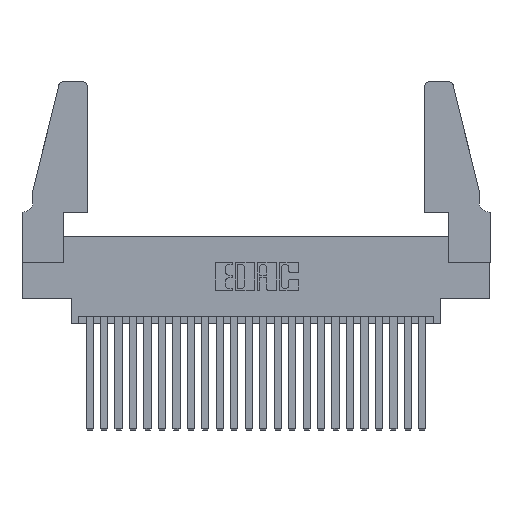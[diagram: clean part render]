
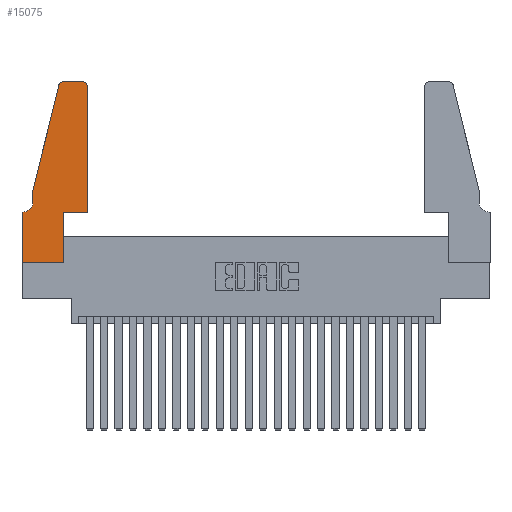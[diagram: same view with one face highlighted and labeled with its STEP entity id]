
A CAD part, top view. The second image highlights one B-rep face of the part: STEP entity #15075.
In plain terms, the highlighted planar face has unit normal (0, 0, 1).
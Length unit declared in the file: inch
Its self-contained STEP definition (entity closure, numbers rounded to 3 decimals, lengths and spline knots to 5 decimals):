
#36 = CARTESIAN_POINT ( 'NONE',  ( 0.2865, 0., 0.37 ) ) ;
#177 = CARTESIAN_POINT ( 'NONE',  ( 0.4505, 0.35, 0.37 ) ) ;
#179 = DIRECTION ( 'NONE',  ( 1., 0., 0. ) ) ;
#201 = VECTOR ( 'NONE', #4903, 39.37008 ) ;
#260 = DIRECTION ( 'NONE',  ( 0., 0., 1. ) ) ;
#274 = VECTOR ( 'NONE', #13782, 39.37008 ) ;
#281 = CARTESIAN_POINT ( 'NONE',  ( 0.2865, 0.35, 0.37 ) ) ;
#748 = CARTESIAN_POINT ( 'NONE',  ( 0.25487, 1.22718, 0.37 ) ) ;
#783 = EDGE_CURVE ( 'NONE', #15887, #18100, #9554, .T. ) ;
#803 = DIRECTION ( 'NONE',  ( -1., 0., 0. ) ) ;
#973 = VECTOR ( 'NONE', #17176, 39.37008 ) ;
#1058 = CARTESIAN_POINT ( 'NONE',  ( 0.0755, 0.42, 0.37 ) ) ;
#1167 = LINE ( 'NONE', #7243, #19781 ) ;
#1214 = CARTESIAN_POINT ( 'NONE',  ( 0.2865, 0.35, 0.37 ) ) ;
#1981 = ORIENTED_EDGE ( 'NONE', *, *, #14536, .T. ) ;
#2157 = LINE ( 'NONE', #17942, #21330 ) ;
#2161 = CARTESIAN_POINT ( 'NONE',  ( 0., 0., 0.37 ) ) ;
#2230 = CARTESIAN_POINT ( 'NONE',  ( 0., 0.35, 0.37 ) ) ;
#2284 = VERTEX_POINT ( 'NONE', #1058 ) ;
#2475 = ORIENTED_EDGE ( 'NONE', *, *, #21416, .T. ) ;
#2632 = DIRECTION ( 'NONE',  ( 0., 0., 1. ) ) ;
#2735 = CARTESIAN_POINT ( 'NONE',  ( 0.0755, 0.35, 0.37 ) ) ;
#2858 = EDGE_CURVE ( 'NONE', #8271, #17694, #12564, .T. ) ;
#2925 = DIRECTION ( 'NONE',  ( -1., 0., 0. ) ) ;
#2994 = ORIENTED_EDGE ( 'NONE', *, *, #15100, .T. ) ;
#3627 = CARTESIAN_POINT ( 'NONE',  ( 0.4205, 1.25, 0.37 ) ) ;
#3668 = DIRECTION ( 'NONE',  ( 0., -1., 0. ) ) ;
#3981 = CARTESIAN_POINT ( 'NONE',  ( 0.4505, 0.35, 0.37 ) ) ;
#4006 = ORIENTED_EDGE ( 'NONE', *, *, #16755, .T. ) ;
#4369 = LINE ( 'NONE', #20888, #9184 ) ;
#4506 = ORIENTED_EDGE ( 'NONE', *, *, #20100, .T. ) ;
#4723 = VERTEX_POINT ( 'NONE', #20505 ) ;
#4899 = LINE ( 'NONE', #2161, #13919 ) ;
#4903 = DIRECTION ( 'NONE',  ( 0., 1., 0. ) ) ;
#5334 = VECTOR ( 'NONE', #10659, 39.37008 ) ;
#5396 = PLANE ( 'NONE',  #8343 ) ;
#7199 = DIRECTION ( 'NONE',  ( 0., 0., 1. ) ) ;
#7243 = CARTESIAN_POINT ( 'NONE',  ( 0.0755, 0.5, 0.37 ) ) ;
#7480 = VERTEX_POINT ( 'NONE', #21115 ) ;
#7668 = DIRECTION ( 'NONE',  ( 1., 0., 0. ) ) ;
#8141 = ORIENTED_EDGE ( 'NONE', *, *, #18767, .T. ) ;
#8268 = VERTEX_POINT ( 'NONE', #281 ) ;
#8271 = VERTEX_POINT ( 'NONE', #9369 ) ;
#8343 = AXIS2_PLACEMENT_3D ( 'NONE', #12489, #7199, #19747 ) ;
#8562 = EDGE_CURVE ( 'NONE', #8845, #8271, #4369, .T. ) ;
#8845 = VERTEX_POINT ( 'NONE', #3627 ) ;
#9036 = CARTESIAN_POINT ( 'NONE',  ( 0.4505, 1.22, 0.37 ) ) ;
#9133 = EDGE_CURVE ( 'NONE', #2284, #7480, #18961, .T. ) ;
#9184 = VECTOR ( 'NONE', #2925, 39.37008 ) ;
#9369 = CARTESIAN_POINT ( 'NONE',  ( 0.284, 1.25, 0.37 ) ) ;
#9376 = ORIENTED_EDGE ( 'NONE', *, *, #783, .T. ) ;
#9554 = LINE ( 'NONE', #177, #5334 ) ;
#9665 = VERTEX_POINT ( 'NONE', #2230 ) ;
#10659 = DIRECTION ( 'NONE',  ( 0., 1., 0. ) ) ;
#11168 = CARTESIAN_POINT ( 'NONE',  ( 0.4205, 1.22, 0.37 ) ) ;
#11707 = DIRECTION ( 'NONE',  ( 0., 0., -1. ) ) ;
#11806 = CARTESIAN_POINT ( 'NONE',  ( 0.0755, 0.5, 0.37 ) ) ;
#11965 = EDGE_LOOP ( 'NONE', ( #22827, #23193, #2475, #17290, #16442, #4006, #2994, #8141, #13435, #1981, #9376, #4506 ) ) ;
#12414 = VERTEX_POINT ( 'NONE', #36 ) ;
#12489 = CARTESIAN_POINT ( 'NONE',  ( 0., 0.35, 0.37 ) ) ;
#12564 = CIRCLE ( 'NONE', #16570, 0.03 ) ;
#12896 = CARTESIAN_POINT ( 'NONE',  ( 0.4505, 0.35, 0.37 ) ) ;
#12964 = DIRECTION ( 'NONE',  ( 1., 0., 0. ) ) ;
#13435 = ORIENTED_EDGE ( 'NONE', *, *, #22760, .T. ) ;
#13479 = CARTESIAN_POINT ( 'NONE',  ( 0.284, 1.22, 0.37 ) ) ;
#13782 = DIRECTION ( 'NONE',  ( -0.239, -0.971, 0. ) ) ;
#13919 = VECTOR ( 'NONE', #7668, 39.37008 ) ;
#14263 = LINE ( 'NONE', #12896, #22093 ) ;
#14536 = EDGE_CURVE ( 'NONE', #8268, #15887, #14263, .T. ) ;
#15075 = ADVANCED_FACE ( 'NONE', ( #17132 ), #5396, .T. ) ;
#15100 = EDGE_CURVE ( 'NONE', #9665, #4723, #2157, .T. ) ;
#15277 = DIRECTION ( 'NONE',  ( 1., 0., 0. ) ) ;
#15887 = VERTEX_POINT ( 'NONE', #3981 ) ;
#16442 = ORIENTED_EDGE ( 'NONE', *, *, #9133, .T. ) ;
#16570 = AXIS2_PLACEMENT_3D ( 'NONE', #13479, #2632, #15277 ) ;
#16755 = EDGE_CURVE ( 'NONE', #7480, #9665, #19603, .T. ) ;
#17132 = FACE_OUTER_BOUND ( 'NONE', #11965, .T. ) ;
#17176 = DIRECTION ( 'NONE',  ( -1., 0., 0. ) ) ;
#17290 = ORIENTED_EDGE ( 'NONE', *, *, #21133, .T. ) ;
#17694 = VERTEX_POINT ( 'NONE', #748 ) ;
#17764 = VERTEX_POINT ( 'NONE', #11806 ) ;
#17942 = CARTESIAN_POINT ( 'NONE',  ( 0., 0., 0.37 ) ) ;
#18100 = VERTEX_POINT ( 'NONE', #9036 ) ;
#18767 = EDGE_CURVE ( 'NONE', #4723, #12414, #4899, .T. ) ;
#18961 = CIRCLE ( 'NONE', #20099, 0.07 ) ;
#19165 = CIRCLE ( 'NONE', #21550, 0.03 ) ;
#19435 = LINE ( 'NONE', #1214, #201 ) ;
#19500 = LINE ( 'NONE', #22712, #274 ) ;
#19603 = LINE ( 'NONE', #2735, #973 ) ;
#19747 = DIRECTION ( 'NONE',  ( 1., 0., 0. ) ) ;
#19781 = VECTOR ( 'NONE', #3668, 39.37008 ) ;
#20099 = AXIS2_PLACEMENT_3D ( 'NONE', #22429, #11707, #803 ) ;
#20100 = EDGE_CURVE ( 'NONE', #18100, #8845, #19165, .T. ) ;
#20505 = CARTESIAN_POINT ( 'NONE',  ( 0., 0., 0.37 ) ) ;
#20888 = CARTESIAN_POINT ( 'NONE',  ( 0.2605, 1.25, 0.37 ) ) ;
#21115 = CARTESIAN_POINT ( 'NONE',  ( 0.0055, 0.35, 0.37 ) ) ;
#21133 = EDGE_CURVE ( 'NONE', #17764, #2284, #1167, .T. ) ;
#21330 = VECTOR ( 'NONE', #23353, 39.37008 ) ;
#21416 = EDGE_CURVE ( 'NONE', #17694, #17764, #19500, .T. ) ;
#21550 = AXIS2_PLACEMENT_3D ( 'NONE', #11168, #260, #12964 ) ;
#22093 = VECTOR ( 'NONE', #179, 39.37008 ) ;
#22429 = CARTESIAN_POINT ( 'NONE',  ( 0.0055, 0.42, 0.37 ) ) ;
#22712 = CARTESIAN_POINT ( 'NONE',  ( 0.0755, 0.5, 0.37 ) ) ;
#22760 = EDGE_CURVE ( 'NONE', #12414, #8268, #19435, .T. ) ;
#22827 = ORIENTED_EDGE ( 'NONE', *, *, #8562, .T. ) ;
#23193 = ORIENTED_EDGE ( 'NONE', *, *, #2858, .T. ) ;
#23353 = DIRECTION ( 'NONE',  ( 0., -1., 0. ) ) ;
